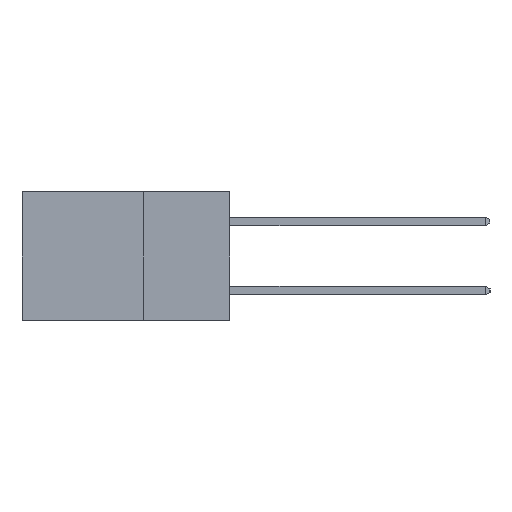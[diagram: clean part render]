
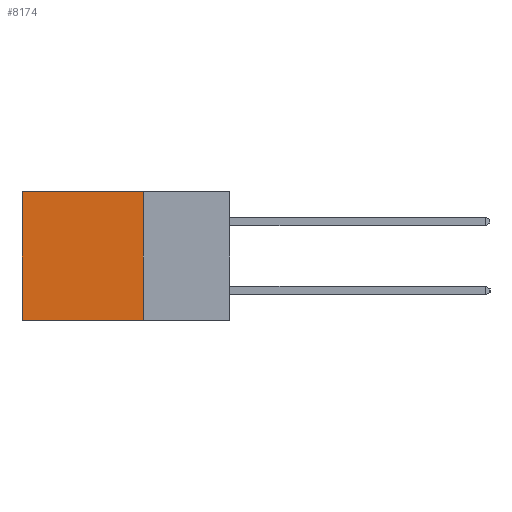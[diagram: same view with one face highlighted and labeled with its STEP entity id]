
A CAD part, left-side view. The second image highlights one B-rep face of the part: STEP entity #8174.
In plain terms, the highlighted planar face has unit normal (-1, 0, 0).
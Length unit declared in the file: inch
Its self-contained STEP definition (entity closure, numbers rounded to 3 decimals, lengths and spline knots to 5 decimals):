
#294 = DIRECTION ( 'NONE',  ( 0., 1., 0. ) ) ;
#590 = CARTESIAN_POINT ( 'NONE',  ( 0.2615, 0.6, -0.37 ) ) ;
#1340 = ORIENTED_EDGE ( 'NONE', *, *, #12461, .T. ) ;
#1647 = EDGE_CURVE ( 'NONE', #19617, #12007, #19142, .T. ) ;
#1812 = DIRECTION ( 'NONE',  ( 0., 0., -1. ) ) ;
#2271 = CARTESIAN_POINT ( 'NONE',  ( 0.2615, 0.6, 0. ) ) ;
#2420 = DIRECTION ( 'NONE',  ( 0., 0., -1. ) ) ;
#2859 = VECTOR ( 'NONE', #2420, 39.37008 ) ;
#4319 = EDGE_LOOP ( 'NONE', ( #1340, #18695, #13608, #11201 ) ) ;
#5614 = DIRECTION ( 'NONE',  ( 0., 0., -1. ) ) ;
#5744 = VECTOR ( 'NONE', #294, 39.37008 ) ;
#6033 = CARTESIAN_POINT ( 'NONE',  ( 0.2615, 0.25, 0. ) ) ;
#8174 = ADVANCED_FACE ( 'NONE', ( #17590 ), #21270, .F. ) ;
#9271 = LINE ( 'NONE', #19828, #18169 ) ;
#9747 = EDGE_CURVE ( 'NONE', #21318, #20082, #10559, .T. ) ;
#10369 = DIRECTION ( 'NONE',  ( 0., 1., 0. ) ) ;
#10421 = CARTESIAN_POINT ( 'NONE',  ( 0.2615, 0.25, -0.37 ) ) ;
#10559 = LINE ( 'NONE', #19905, #5744 ) ;
#10764 = CARTESIAN_POINT ( 'NONE',  ( 0.2615, 0.25, -0.37 ) ) ;
#11201 = ORIENTED_EDGE ( 'NONE', *, *, #9747, .T. ) ;
#12007 = VERTEX_POINT ( 'NONE', #15083 ) ;
#12461 = EDGE_CURVE ( 'NONE', #20082, #12007, #16508, .T. ) ;
#12550 = DIRECTION ( 'NONE',  ( 1., 0., 0. ) ) ;
#13608 = ORIENTED_EDGE ( 'NONE', *, *, #17589, .F. ) ;
#14439 = VECTOR ( 'NONE', #10369, 39.37008 ) ;
#15083 = CARTESIAN_POINT ( 'NONE',  ( 0.2615, 0.6, -0.37 ) ) ;
#16508 = LINE ( 'NONE', #590, #2859 ) ;
#17123 = CARTESIAN_POINT ( 'NONE',  ( 0.2615, 0.25, -0.37 ) ) ;
#17589 = EDGE_CURVE ( 'NONE', #21318, #19617, #9271, .T. ) ;
#17590 = FACE_OUTER_BOUND ( 'NONE', #4319, .T. ) ;
#18169 = VECTOR ( 'NONE', #5614, 39.37008 ) ;
#18695 = ORIENTED_EDGE ( 'NONE', *, *, #1647, .F. ) ;
#19142 = LINE ( 'NONE', #10421, #14439 ) ;
#19617 = VERTEX_POINT ( 'NONE', #17123 ) ;
#19828 = CARTESIAN_POINT ( 'NONE',  ( 0.2615, 0.25, -0.37 ) ) ;
#19905 = CARTESIAN_POINT ( 'NONE',  ( 0.2615, 0.25, 0. ) ) ;
#20082 = VERTEX_POINT ( 'NONE', #2271 ) ;
#20797 = AXIS2_PLACEMENT_3D ( 'NONE', #10764, #12550, #1812 ) ;
#21270 = PLANE ( 'NONE',  #20797 ) ;
#21318 = VERTEX_POINT ( 'NONE', #6033 ) ;
